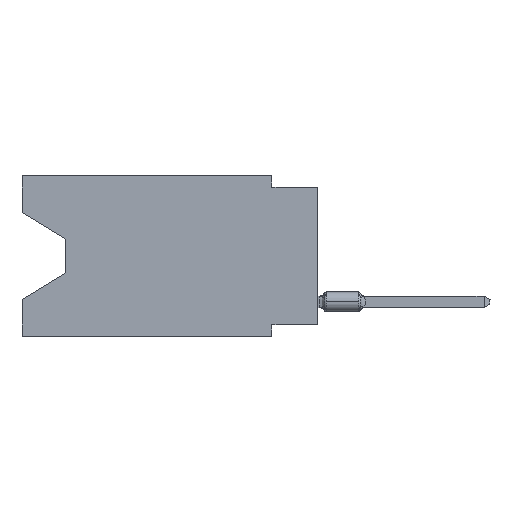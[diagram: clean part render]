
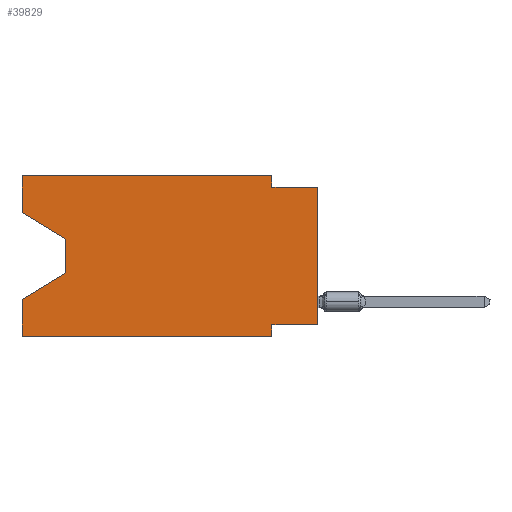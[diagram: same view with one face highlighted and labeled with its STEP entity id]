
A CAD part, left-side view. The second image highlights one B-rep face of the part: STEP entity #39829.
In plain terms, the highlighted planar face has unit normal (-1, 0, 0).
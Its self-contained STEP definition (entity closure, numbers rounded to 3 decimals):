
#1345 = ORIENTED_EDGE ( 'NONE', *, *, #9326, .T. ) ;
#1947 = VECTOR ( 'NONE', #17688, 1000. ) ;
#2432 = CARTESIAN_POINT ( 'NONE',  ( 0., 16.383, 0. ) ) ;
#3046 = CARTESIAN_POINT ( 'NONE',  ( 0., 2.54, -8.89 ) ) ;
#3922 = PLANE ( 'NONE',  #34081 ) ;
#5978 = CARTESIAN_POINT ( 'NONE',  ( 0., 16.383, -2.038 ) ) ;
#6386 = CARTESIAN_POINT ( 'NONE',  ( 0., 13.97, -5.385 ) ) ;
#6863 = EDGE_CURVE ( 'NONE', #46331, #17716, #16564, .T. ) ;
#7346 = DIRECTION ( 'NONE',  ( 0., -0.855, -0.519 ) ) ;
#7893 = ORIENTED_EDGE ( 'NONE', *, *, #43687, .F. ) ;
#8187 = VECTOR ( 'NONE', #38036, 1000. ) ;
#8376 = LINE ( 'NONE', #41951, #38667 ) ;
#9087 = CARTESIAN_POINT ( 'NONE',  ( 0., 13.97, -3.505 ) ) ;
#9326 = EDGE_CURVE ( 'NONE', #52416, #26451, #22921, .T. ) ;
#9736 = CARTESIAN_POINT ( 'NONE',  ( 0., 0., -0.635 ) ) ;
#9873 = DIRECTION ( 'NONE',  ( 0., 0.855, -0.519 ) ) ;
#10115 = ORIENTED_EDGE ( 'NONE', *, *, #33788, .T. ) ;
#12313 = CARTESIAN_POINT ( 'NONE',  ( 0., 0., -0.635 ) ) ;
#12888 = VECTOR ( 'NONE', #25069, 1000. ) ;
#13480 = CARTESIAN_POINT ( 'NONE',  ( 0., 2.54, -0.635 ) ) ;
#13973 = CARTESIAN_POINT ( 'NONE',  ( 0., 0., -8.255 ) ) ;
#14899 = VERTEX_POINT ( 'NONE', #13480 ) ;
#16038 = VERTEX_POINT ( 'NONE', #39596 ) ;
#16475 = EDGE_CURVE ( 'NONE', #16038, #18072, #31080, .T. ) ;
#16564 = LINE ( 'NONE', #25593, #23575 ) ;
#16710 = EDGE_CURVE ( 'NONE', #46331, #16038, #33845, .T. ) ;
#17688 = DIRECTION ( 'NONE',  ( 0., -1., 0. ) ) ;
#17716 = VERTEX_POINT ( 'NONE', #2432 ) ;
#18072 = VERTEX_POINT ( 'NONE', #6386 ) ;
#18280 = LINE ( 'NONE', #52104, #40354 ) ;
#18464 = CARTESIAN_POINT ( 'NONE',  ( 0., 2.54, -8.255 ) ) ;
#19495 = VERTEX_POINT ( 'NONE', #18464 ) ;
#19786 = ORIENTED_EDGE ( 'NONE', *, *, #16710, .T. ) ;
#20260 = DIRECTION ( 'NONE',  ( 0., 0., -1. ) ) ;
#20552 = LINE ( 'NONE', #37738, #12888 ) ;
#21137 = CARTESIAN_POINT ( 'NONE',  ( 0., 16.383, 0. ) ) ;
#22430 = VERTEX_POINT ( 'NONE', #48347 ) ;
#22608 = EDGE_LOOP ( 'NONE', ( #19786, #24187, #10115, #7893, #1345, #43834, #48601, #41035, #39498, #45381, #43442, #31727 ) ) ;
#22921 = LINE ( 'NONE', #35594, #26670 ) ;
#22953 = CARTESIAN_POINT ( 'NONE',  ( 0., 16.383, -8.89 ) ) ;
#23575 = VECTOR ( 'NONE', #30647, 1000. ) ;
#24187 = ORIENTED_EDGE ( 'NONE', *, *, #16475, .T. ) ;
#25040 = LINE ( 'NONE', #12313, #1947 ) ;
#25069 = DIRECTION ( 'NONE',  ( 0., -1., 0. ) ) ;
#25342 = VECTOR ( 'NONE', #7346, 1000. ) ;
#25580 = EDGE_CURVE ( 'NONE', #22430, #14899, #51089, .T. ) ;
#25593 = CARTESIAN_POINT ( 'NONE',  ( 0., 16.383, 0. ) ) ;
#26310 = DIRECTION ( 'NONE',  ( 0., 0., -1. ) ) ;
#26431 = EDGE_CURVE ( 'NONE', #52577, #19495, #8376, .T. ) ;
#26451 = VERTEX_POINT ( 'NONE', #42793 ) ;
#26670 = VECTOR ( 'NONE', #44886, 1000. ) ;
#26759 = VECTOR ( 'NONE', #9873, 1000. ) ;
#27386 = LINE ( 'NONE', #52182, #26759 ) ;
#27428 = VECTOR ( 'NONE', #20260, 1000. ) ;
#27824 = VECTOR ( 'NONE', #47420, 1000. ) ;
#27993 = VECTOR ( 'NONE', #26310, 1000. ) ;
#28710 = LINE ( 'NONE', #3046, #27428 ) ;
#30236 = CARTESIAN_POINT ( 'NONE',  ( 0., 2.54, 0. ) ) ;
#30424 = LINE ( 'NONE', #42828, #8187 ) ;
#30647 = DIRECTION ( 'NONE',  ( 0., 0., 1. ) ) ;
#31080 = LINE ( 'NONE', #9087, #27993 ) ;
#31727 = ORIENTED_EDGE ( 'NONE', *, *, #6863, .F. ) ;
#33788 = EDGE_CURVE ( 'NONE', #18072, #34239, #27386, .T. ) ;
#33845 = LINE ( 'NONE', #42029, #25342 ) ;
#34081 = AXIS2_PLACEMENT_3D ( 'NONE', #21137, #38313, #55771 ) ;
#34239 = VERTEX_POINT ( 'NONE', #44429 ) ;
#34244 = VERTEX_POINT ( 'NONE', #9736 ) ;
#34652 = FACE_OUTER_BOUND ( 'NONE', #22608, .T. ) ;
#35594 = CARTESIAN_POINT ( 'NONE',  ( 0., 16.383, -8.89 ) ) ;
#37738 = CARTESIAN_POINT ( 'NONE',  ( 0., 16.383, 0. ) ) ;
#38036 = DIRECTION ( 'NONE',  ( 0., 0., 1. ) ) ;
#38313 = DIRECTION ( 'NONE',  ( 1., 0., 0. ) ) ;
#38667 = VECTOR ( 'NONE', #42516, 1000. ) ;
#39498 = ORIENTED_EDGE ( 'NONE', *, *, #54372, .F. ) ;
#39596 = CARTESIAN_POINT ( 'NONE',  ( 0., 13.97, -3.505 ) ) ;
#39829 = ADVANCED_FACE ( 'NONE', ( #34652 ), #3922, .F. ) ;
#40354 = VECTOR ( 'NONE', #44480, 1000. ) ;
#41035 = ORIENTED_EDGE ( 'NONE', *, *, #41327, .T. ) ;
#41327 = EDGE_CURVE ( 'NONE', #52577, #34244, #30424, .T. ) ;
#41951 = CARTESIAN_POINT ( 'NONE',  ( 0., 0., -8.255 ) ) ;
#42029 = CARTESIAN_POINT ( 'NONE',  ( 0., 16.383, -2.038 ) ) ;
#42516 = DIRECTION ( 'NONE',  ( 0., 1., 0. ) ) ;
#42793 = CARTESIAN_POINT ( 'NONE',  ( 0., 2.54, -8.89 ) ) ;
#42828 = CARTESIAN_POINT ( 'NONE',  ( 0., 0., 0. ) ) ;
#43442 = ORIENTED_EDGE ( 'NONE', *, *, #45375, .F. ) ;
#43687 = EDGE_CURVE ( 'NONE', #52416, #34239, #18280, .T. ) ;
#43834 = ORIENTED_EDGE ( 'NONE', *, *, #47145, .F. ) ;
#44429 = CARTESIAN_POINT ( 'NONE',  ( 0., 16.383, -6.852 ) ) ;
#44480 = DIRECTION ( 'NONE',  ( 0., 0., 1. ) ) ;
#44886 = DIRECTION ( 'NONE',  ( 0., -1., 0. ) ) ;
#45375 = EDGE_CURVE ( 'NONE', #17716, #22430, #20552, .T. ) ;
#45381 = ORIENTED_EDGE ( 'NONE', *, *, #25580, .F. ) ;
#46331 = VERTEX_POINT ( 'NONE', #5978 ) ;
#47145 = EDGE_CURVE ( 'NONE', #19495, #26451, #28710, .T. ) ;
#47420 = DIRECTION ( 'NONE',  ( 0., 0., -1. ) ) ;
#48347 = CARTESIAN_POINT ( 'NONE',  ( 0., 2.54, 0. ) ) ;
#48601 = ORIENTED_EDGE ( 'NONE', *, *, #26431, .F. ) ;
#51089 = LINE ( 'NONE', #30236, #27824 ) ;
#52104 = CARTESIAN_POINT ( 'NONE',  ( 0., 16.383, 0. ) ) ;
#52182 = CARTESIAN_POINT ( 'NONE',  ( 0., 13.97, -5.385 ) ) ;
#52416 = VERTEX_POINT ( 'NONE', #22953 ) ;
#52577 = VERTEX_POINT ( 'NONE', #13973 ) ;
#54372 = EDGE_CURVE ( 'NONE', #14899, #34244, #25040, .T. ) ;
#55771 = DIRECTION ( 'NONE',  ( 0., 0., -1. ) ) ;
